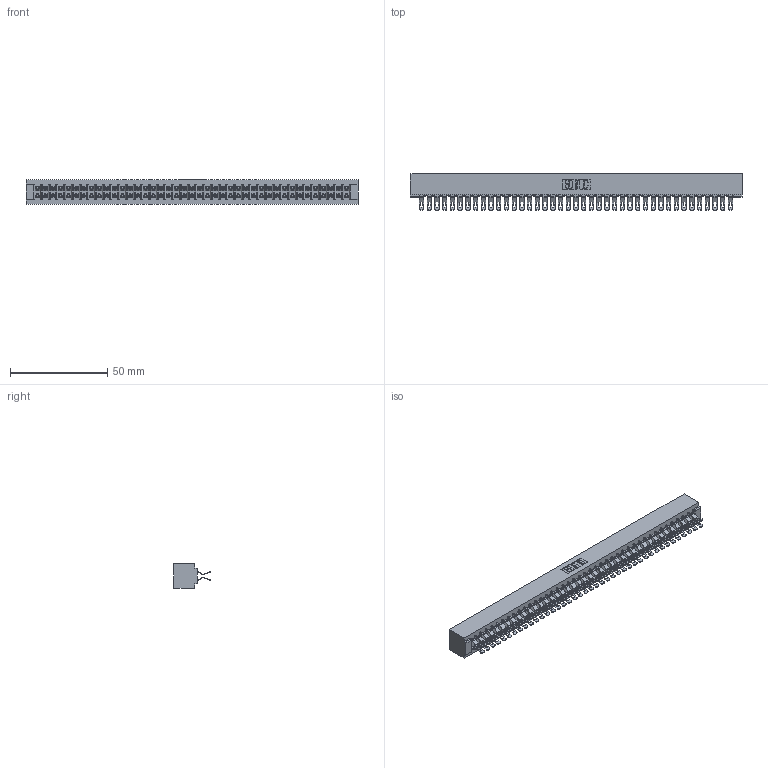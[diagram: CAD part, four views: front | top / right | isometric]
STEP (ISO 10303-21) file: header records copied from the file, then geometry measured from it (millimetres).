
FILE_DESCRIPTION (( 'STEP AP203' ), '1' );
FILE_NAME ('357-082-455-201.STEP', '2020-10-04T09:43:42', ( '' ), ( '' ), 'SwSTEP 2.0', 'SolidWorks 2020', '' );
FILE_SCHEMA (( 'CONFIG_CONTROL_DESIGN' ));
Length unit declared in the file: inch
Products named in the file (3): 357-082-455-201; 307-290-001_555; 307 Part_No Mounting Lugs
Assembly tree (83 placements, depth 2):
  357-082-455-201
    307 Part_No Mounting Lugs
    307-290-001_555  x82
Bounding box: 170.33 x 18.75 x 12.7 mm (x, y, z)
Volume: 18897.6 mm3; surface area: 24773 mm2
Topology: 83 solids, 83 shells, 5154 faces, 15141 edges, 9870 vertices
Faces by surface type: plane 2854, cylinder 2216, sphere 84
Entity records: 36843 total; most frequent: CARTESIAN_POINT 6029, ORIENTED_EDGE 5976, DIRECTION 5912, EDGE_CURVE 2988, LINE 2282, VECTOR 2282, VERTEX_POINT 1932, AXIS2_PLACEMENT_3D 1815
